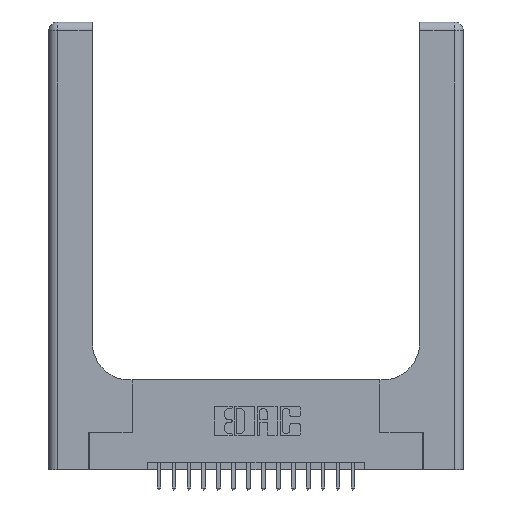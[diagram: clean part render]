
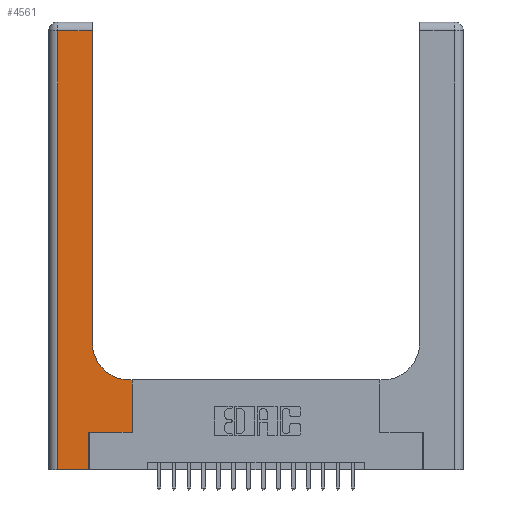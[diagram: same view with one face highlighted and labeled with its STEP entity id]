
A CAD part, top view. The second image highlights one B-rep face of the part: STEP entity #4561.
In plain terms, the highlighted planar face has unit normal (0, 0, 1).
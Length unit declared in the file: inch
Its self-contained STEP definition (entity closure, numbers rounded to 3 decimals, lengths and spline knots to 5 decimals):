
#22 = CARTESIAN_POINT ( 'NONE',  ( 0.06, 2.94, 0.37 ) ) ;
#141 = ORIENTED_EDGE ( 'NONE', *, *, #6676, .T. ) ;
#189 = VECTOR ( 'NONE', #3862, 39.37008 ) ;
#535 = LINE ( 'NONE', #16292, #9326 ) ;
#999 = DIRECTION ( 'NONE',  ( 0., 0., -1. ) ) ;
#1009 = EDGE_CURVE ( 'NONE', #4327, #2445, #4443, .T. ) ;
#1083 = CIRCLE ( 'NONE', #13846, 0.25 ) ;
#1086 = CARTESIAN_POINT ( 'NONE',  ( 0.2915, 0.6, 0.37 ) ) ;
#1319 = DIRECTION ( 'NONE',  ( 1., 0., 0. ) ) ;
#1360 = LINE ( 'NONE', #10346, #12724 ) ;
#2202 = LINE ( 'NONE', #17130, #19034 ) ;
#2380 = LINE ( 'NONE', #2384, #10137 ) ;
#2384 = CARTESIAN_POINT ( 'NONE',  ( 0.269, 0.25, 0.37 ) ) ;
#2435 = VERTEX_POINT ( 'NONE', #15377 ) ;
#2445 = VERTEX_POINT ( 'NONE', #18260 ) ;
#2585 = FACE_OUTER_BOUND ( 'NONE', #8262, .T. ) ;
#2596 = VERTEX_POINT ( 'NONE', #11204 ) ;
#3303 = EDGE_CURVE ( 'NONE', #2435, #11958, #3397, .T. ) ;
#3310 = DIRECTION ( 'NONE',  ( 1., 0., 0. ) ) ;
#3397 = LINE ( 'NONE', #10953, #19199 ) ;
#3862 = DIRECTION ( 'NONE',  ( 0., 1., 0. ) ) ;
#3943 = AXIS2_PLACEMENT_3D ( 'NONE', #5699, #999, #11843 ) ;
#4003 = DIRECTION ( 'NONE',  ( 1., 0., 0. ) ) ;
#4088 = EDGE_CURVE ( 'NONE', #11958, #18032, #18942, .T. ) ;
#4256 = LINE ( 'NONE', #7067, #15045 ) ;
#4327 = VERTEX_POINT ( 'NONE', #4756 ) ;
#4351 = VERTEX_POINT ( 'NONE', #22 ) ;
#4443 = LINE ( 'NONE', #15264, #189 ) ;
#4561 = ADVANCED_FACE ( 'NONE', ( #2585 ), #19424, .F. ) ;
#4756 = CARTESIAN_POINT ( 'NONE',  ( 0.2915, 0.85, 0.37 ) ) ;
#5146 = EDGE_CURVE ( 'NONE', #18032, #4327, #1083, .T. ) ;
#5699 = CARTESIAN_POINT ( 'NONE',  ( 0., 3., 0.37 ) ) ;
#6676 = EDGE_CURVE ( 'NONE', #4351, #10436, #4256, .T. ) ;
#6874 = ORIENTED_EDGE ( 'NONE', *, *, #9366, .T. ) ;
#7067 = CARTESIAN_POINT ( 'NONE',  ( 0.06, 3., 0.37 ) ) ;
#7105 = DIRECTION ( 'NONE',  ( -1., 0., 0. ) ) ;
#7652 = ORIENTED_EDGE ( 'NONE', *, *, #3303, .T. ) ;
#7728 = ORIENTED_EDGE ( 'NONE', *, *, #14154, .T. ) ;
#8262 = EDGE_LOOP ( 'NONE', ( #10508, #16637, #141, #19627, #6874, #7728, #7652, #10054, #11840 ) ) ;
#9326 = VECTOR ( 'NONE', #7105, 39.37008 ) ;
#9366 = EDGE_CURVE ( 'NONE', #12679, #2596, #1360, .T. ) ;
#10054 = ORIENTED_EDGE ( 'NONE', *, *, #4088, .T. ) ;
#10137 = VECTOR ( 'NONE', #4003, 39.37008 ) ;
#10346 = CARTESIAN_POINT ( 'NONE',  ( 0.269, 0., 0.37 ) ) ;
#10390 = DIRECTION ( 'NONE',  ( -1., 0., 0. ) ) ;
#10436 = VERTEX_POINT ( 'NONE', #14791 ) ;
#10508 = ORIENTED_EDGE ( 'NONE', *, *, #1009, .T. ) ;
#10615 = DIRECTION ( 'NONE',  ( 0., 0., -1. ) ) ;
#10714 = DIRECTION ( 'NONE',  ( 0., 1., 0. ) ) ;
#10953 = CARTESIAN_POINT ( 'NONE',  ( 0.5585, 0.25, 0.37 ) ) ;
#11204 = CARTESIAN_POINT ( 'NONE',  ( 0.269, 0.25, 0.37 ) ) ;
#11840 = ORIENTED_EDGE ( 'NONE', *, *, #5146, .T. ) ;
#11843 = DIRECTION ( 'NONE',  ( -1., 0., 0. ) ) ;
#11958 = VERTEX_POINT ( 'NONE', #16947 ) ;
#12545 = EDGE_CURVE ( 'NONE', #10436, #12679, #2202, .T. ) ;
#12679 = VERTEX_POINT ( 'NONE', #17393 ) ;
#12724 = VECTOR ( 'NONE', #17964, 39.37008 ) ;
#13846 = AXIS2_PLACEMENT_3D ( 'NONE', #19726, #10615, #1319 ) ;
#14154 = EDGE_CURVE ( 'NONE', #2596, #2435, #2380, .T. ) ;
#14620 = CARTESIAN_POINT ( 'NONE',  ( 0.5415, 0.6, 0.37 ) ) ;
#14791 = CARTESIAN_POINT ( 'NONE',  ( 0.06, 0., 0.37 ) ) ;
#15045 = VECTOR ( 'NONE', #17776, 39.37008 ) ;
#15264 = CARTESIAN_POINT ( 'NONE',  ( 0.2915, 3., 0.37 ) ) ;
#15377 = CARTESIAN_POINT ( 'NONE',  ( 0.5585, 0.25, 0.37 ) ) ;
#16292 = CARTESIAN_POINT ( 'NONE',  ( 0., 2.94, 0.37 ) ) ;
#16637 = ORIENTED_EDGE ( 'NONE', *, *, #18463, .T. ) ;
#16947 = CARTESIAN_POINT ( 'NONE',  ( 0.5585, 0.6, 0.37 ) ) ;
#17130 = CARTESIAN_POINT ( 'NONE',  ( 0., 0., 0.37 ) ) ;
#17393 = CARTESIAN_POINT ( 'NONE',  ( 0.269, 0., 0.37 ) ) ;
#17776 = DIRECTION ( 'NONE',  ( 0., -1., 0. ) ) ;
#17964 = DIRECTION ( 'NONE',  ( 0., 1., 0. ) ) ;
#18032 = VERTEX_POINT ( 'NONE', #14620 ) ;
#18260 = CARTESIAN_POINT ( 'NONE',  ( 0.2915, 2.94, 0.37 ) ) ;
#18463 = EDGE_CURVE ( 'NONE', #2445, #4351, #535, .T. ) ;
#18487 = VECTOR ( 'NONE', #10390, 39.37008 ) ;
#18942 = LINE ( 'NONE', #1086, #18487 ) ;
#19034 = VECTOR ( 'NONE', #3310, 39.37008 ) ;
#19199 = VECTOR ( 'NONE', #10714, 39.37008 ) ;
#19424 = PLANE ( 'NONE',  #3943 ) ;
#19627 = ORIENTED_EDGE ( 'NONE', *, *, #12545, .T. ) ;
#19726 = CARTESIAN_POINT ( 'NONE',  ( 0.5415, 0.85, 0.37 ) ) ;
